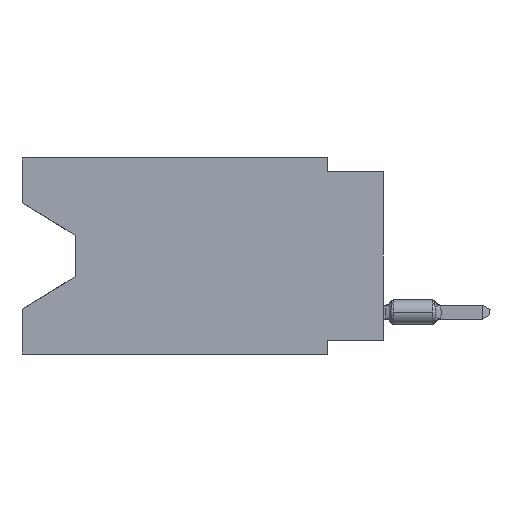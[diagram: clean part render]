
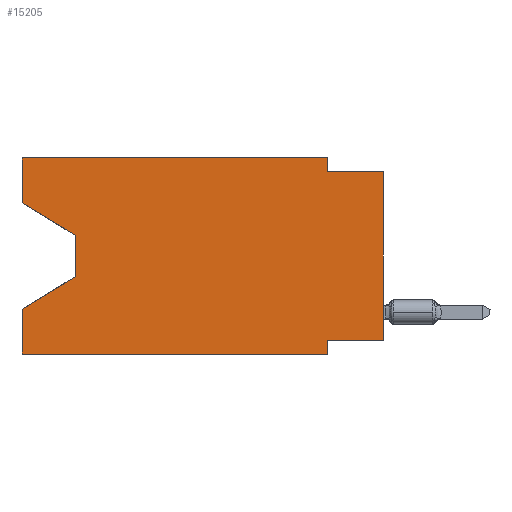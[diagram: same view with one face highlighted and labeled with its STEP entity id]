
A CAD part, left-side view. The second image highlights one B-rep face of the part: STEP entity #15205.
In plain terms, the highlighted planar face has unit normal (-1, 0, 0).
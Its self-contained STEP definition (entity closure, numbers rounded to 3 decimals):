
#19 = EDGE_CURVE ( 'NONE', #11300, #2317, #4853, .T. ) ;
#368 = CARTESIAN_POINT ( 'NONE',  ( 0., 0., -8.255 ) ) ;
#651 = DIRECTION ( 'NONE',  ( 0., -1., 0. ) ) ;
#862 = DIRECTION ( 'NONE',  ( 0., -1., 0. ) ) ;
#972 = ORIENTED_EDGE ( 'NONE', *, *, #7740, .T. ) ;
#1625 = DIRECTION ( 'NONE',  ( 0., 0., 1. ) ) ;
#1636 = CARTESIAN_POINT ( 'NONE',  ( 0., 0., -0.635 ) ) ;
#1918 = LINE ( 'NONE', #7923, #18440 ) ;
#2317 = VERTEX_POINT ( 'NONE', #8172 ) ;
#2382 = LINE ( 'NONE', #18983, #16718 ) ;
#3016 = DIRECTION ( 'NONE',  ( 0., 0., 1. ) ) ;
#3081 = CARTESIAN_POINT ( 'NONE',  ( 0., 16.383, -8.89 ) ) ;
#3340 = CARTESIAN_POINT ( 'NONE',  ( 0., 16.383, 0. ) ) ;
#3389 = EDGE_CURVE ( 'NONE', #15033, #6840, #21903, .T. ) ;
#3730 = CARTESIAN_POINT ( 'NONE',  ( 0., 2.54, -8.89 ) ) ;
#3896 = VECTOR ( 'NONE', #13792, 1000. ) ;
#3976 = EDGE_LOOP ( 'NONE', ( #972, #5944, #5051, #18922, #24243, #6902, #5007, #15634, #10066, #10328, #21100, #12254 ) ) ;
#4249 = VERTEX_POINT ( 'NONE', #5371 ) ;
#4494 = VERTEX_POINT ( 'NONE', #21540 ) ;
#4853 = LINE ( 'NONE', #19845, #20508 ) ;
#4884 = VERTEX_POINT ( 'NONE', #23237 ) ;
#4925 = VECTOR ( 'NONE', #9844, 1000. ) ;
#5007 = ORIENTED_EDGE ( 'NONE', *, *, #16873, .F. ) ;
#5011 = DIRECTION ( 'NONE',  ( 0., -0.855, -0.519 ) ) ;
#5051 = ORIENTED_EDGE ( 'NONE', *, *, #14840, .T. ) ;
#5371 = CARTESIAN_POINT ( 'NONE',  ( 0., 2.54, 0. ) ) ;
#5944 = ORIENTED_EDGE ( 'NONE', *, *, #15413, .T. ) ;
#6169 = CARTESIAN_POINT ( 'NONE',  ( 0., 0., 0. ) ) ;
#6211 = CARTESIAN_POINT ( 'NONE',  ( 0., 16.383, -2.038 ) ) ;
#6642 = EDGE_CURVE ( 'NONE', #6840, #4249, #2382, .T. ) ;
#6760 = LINE ( 'NONE', #3081, #10053 ) ;
#6765 = CARTESIAN_POINT ( 'NONE',  ( 0., 2.54, 0. ) ) ;
#6840 = VERTEX_POINT ( 'NONE', #14909 ) ;
#6902 = ORIENTED_EDGE ( 'NONE', *, *, #20110, .F. ) ;
#6977 = CARTESIAN_POINT ( 'NONE',  ( 0., 13.97, -5.385 ) ) ;
#7162 = EDGE_CURVE ( 'NONE', #11300, #4884, #6760, .T. ) ;
#7740 = EDGE_CURVE ( 'NONE', #15033, #21342, #21845, .T. ) ;
#7892 = CARTESIAN_POINT ( 'NONE',  ( 0., 13.97, -3.505 ) ) ;
#7923 = CARTESIAN_POINT ( 'NONE',  ( 0., 13.97, -5.385 ) ) ;
#8172 = CARTESIAN_POINT ( 'NONE',  ( 0., 16.383, -6.852 ) ) ;
#8248 = DIRECTION ( 'NONE',  ( 0., 0., -1. ) ) ;
#8363 = DIRECTION ( 'NONE',  ( 0., 0., -1. ) ) ;
#8488 = EDGE_CURVE ( 'NONE', #4249, #10481, #14158, .T. ) ;
#8900 = PLANE ( 'NONE',  #11367 ) ;
#9303 = DIRECTION ( 'NONE',  ( 0., 0.855, -0.519 ) ) ;
#9844 = DIRECTION ( 'NONE',  ( 0., 1., 0. ) ) ;
#10053 = VECTOR ( 'NONE', #862, 1000. ) ;
#10066 = ORIENTED_EDGE ( 'NONE', *, *, #13072, .F. ) ;
#10328 = ORIENTED_EDGE ( 'NONE', *, *, #8488, .F. ) ;
#10481 = VERTEX_POINT ( 'NONE', #20455 ) ;
#10869 = FACE_OUTER_BOUND ( 'NONE', #3976, .T. ) ;
#10979 = LINE ( 'NONE', #1636, #18025 ) ;
#11300 = VERTEX_POINT ( 'NONE', #13965 ) ;
#11367 = AXIS2_PLACEMENT_3D ( 'NONE', #20082, #18240, #14687 ) ;
#11380 = VECTOR ( 'NONE', #8248, 1000. ) ;
#12053 = LINE ( 'NONE', #368, #4925 ) ;
#12254 = ORIENTED_EDGE ( 'NONE', *, *, #3389, .F. ) ;
#13072 = EDGE_CURVE ( 'NONE', #10481, #14870, #10979, .T. ) ;
#13081 = DIRECTION ( 'NONE',  ( 0., -1., 0. ) ) ;
#13178 = EDGE_CURVE ( 'NONE', #19470, #14870, #13558, .T. ) ;
#13219 = LINE ( 'NONE', #17722, #11380 ) ;
#13558 = LINE ( 'NONE', #6169, #3896 ) ;
#13792 = DIRECTION ( 'NONE',  ( 0., 0., 1. ) ) ;
#13965 = CARTESIAN_POINT ( 'NONE',  ( 0., 16.383, -8.89 ) ) ;
#14158 = LINE ( 'NONE', #6765, #23431 ) ;
#14687 = DIRECTION ( 'NONE',  ( 0., 0., -1. ) ) ;
#14840 = EDGE_CURVE ( 'NONE', #21972, #2317, #1918, .T. ) ;
#14870 = VERTEX_POINT ( 'NONE', #22315 ) ;
#14909 = CARTESIAN_POINT ( 'NONE',  ( 0., 16.383, 0. ) ) ;
#15033 = VERTEX_POINT ( 'NONE', #6211 ) ;
#15205 = ADVANCED_FACE ( 'NONE', ( #10869 ), #8900, .F. ) ;
#15413 = EDGE_CURVE ( 'NONE', #21342, #21972, #13219, .T. ) ;
#15634 = ORIENTED_EDGE ( 'NONE', *, *, #13178, .T. ) ;
#16718 = VECTOR ( 'NONE', #651, 1000. ) ;
#16873 = EDGE_CURVE ( 'NONE', #19470, #4494, #12053, .T. ) ;
#17722 = CARTESIAN_POINT ( 'NONE',  ( 0., 13.97, -3.505 ) ) ;
#18025 = VECTOR ( 'NONE', #13081, 1000. ) ;
#18212 = VECTOR ( 'NONE', #18966, 1000. ) ;
#18240 = DIRECTION ( 'NONE',  ( 1., 0., 0. ) ) ;
#18285 = CARTESIAN_POINT ( 'NONE',  ( 0., 16.383, -2.038 ) ) ;
#18440 = VECTOR ( 'NONE', #9303, 1000. ) ;
#18922 = ORIENTED_EDGE ( 'NONE', *, *, #19, .F. ) ;
#18966 = DIRECTION ( 'NONE',  ( 0., 0., -1. ) ) ;
#18983 = CARTESIAN_POINT ( 'NONE',  ( 0., 16.383, 0. ) ) ;
#19470 = VERTEX_POINT ( 'NONE', #23429 ) ;
#19845 = CARTESIAN_POINT ( 'NONE',  ( 0., 16.383, 0. ) ) ;
#20082 = CARTESIAN_POINT ( 'NONE',  ( 0., 16.383, 0. ) ) ;
#20110 = EDGE_CURVE ( 'NONE', #4494, #4884, #22773, .T. ) ;
#20455 = CARTESIAN_POINT ( 'NONE',  ( 0., 2.54, -0.635 ) ) ;
#20508 = VECTOR ( 'NONE', #3016, 1000. ) ;
#21100 = ORIENTED_EDGE ( 'NONE', *, *, #6642, .F. ) ;
#21342 = VERTEX_POINT ( 'NONE', #7892 ) ;
#21540 = CARTESIAN_POINT ( 'NONE',  ( 0., 2.54, -8.255 ) ) ;
#21845 = LINE ( 'NONE', #18285, #23007 ) ;
#21903 = LINE ( 'NONE', #3340, #22587 ) ;
#21972 = VERTEX_POINT ( 'NONE', #6977 ) ;
#22315 = CARTESIAN_POINT ( 'NONE',  ( 0., 0., -0.635 ) ) ;
#22587 = VECTOR ( 'NONE', #1625, 1000. ) ;
#22773 = LINE ( 'NONE', #3730, #18212 ) ;
#23007 = VECTOR ( 'NONE', #5011, 1000. ) ;
#23237 = CARTESIAN_POINT ( 'NONE',  ( 0., 2.54, -8.89 ) ) ;
#23429 = CARTESIAN_POINT ( 'NONE',  ( 0., 0., -8.255 ) ) ;
#23431 = VECTOR ( 'NONE', #8363, 1000. ) ;
#24243 = ORIENTED_EDGE ( 'NONE', *, *, #7162, .T. ) ;
